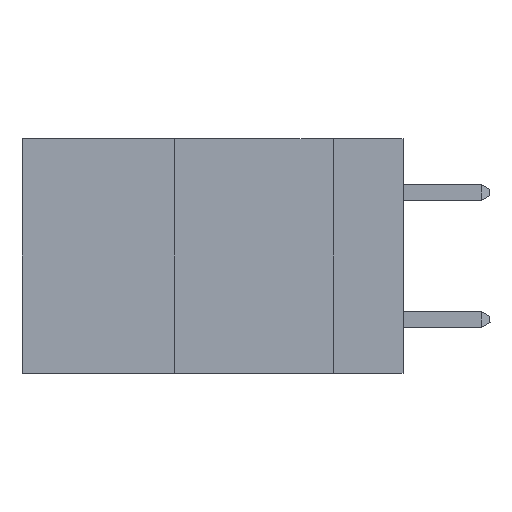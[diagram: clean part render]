
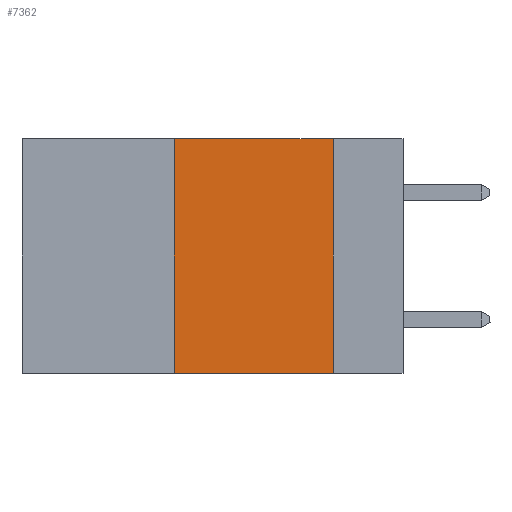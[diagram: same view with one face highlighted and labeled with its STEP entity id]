
A CAD part, left-side view. The second image highlights one B-rep face of the part: STEP entity #7362.
In plain terms, the highlighted planar face has unit normal (-1, 0, 0).
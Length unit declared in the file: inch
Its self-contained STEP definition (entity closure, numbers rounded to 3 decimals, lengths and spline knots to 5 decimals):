
#222 = VERTEX_POINT ( 'NONE', #383 ) ;
#383 = CARTESIAN_POINT ( 'NONE',  ( 0., 0.36, -0.37 ) ) ;
#716 = DIRECTION ( 'NONE',  ( 0., 0., -1. ) ) ;
#1097 = DIRECTION ( 'NONE',  ( 0., 0., 1. ) ) ;
#1168 = VECTOR ( 'NONE', #9938, 39.37008 ) ;
#2051 = CARTESIAN_POINT ( 'NONE',  ( 0., 0.36, 0. ) ) ;
#2286 = CARTESIAN_POINT ( 'NONE',  ( 0., 0.36, 0. ) ) ;
#2443 = EDGE_CURVE ( 'NONE', #222, #6811, #13166, .T. ) ;
#3015 = EDGE_LOOP ( 'NONE', ( #5993, #12001, #3783, #4115 ) ) ;
#3783 = ORIENTED_EDGE ( 'NONE', *, *, #2443, .F. ) ;
#4115 = ORIENTED_EDGE ( 'NONE', *, *, #9766, .T. ) ;
#4386 = LINE ( 'NONE', #5401, #6922 ) ;
#4766 = FACE_OUTER_BOUND ( 'NONE', #3015, .T. ) ;
#5401 = CARTESIAN_POINT ( 'NONE',  ( 0., 0.6, -0.37 ) ) ;
#5694 = CARTESIAN_POINT ( 'NONE',  ( 0., 0.6, 0. ) ) ;
#5993 = ORIENTED_EDGE ( 'NONE', *, *, #7477, .F. ) ;
#6811 = VERTEX_POINT ( 'NONE', #2051 ) ;
#6922 = VECTOR ( 'NONE', #13944, 39.37008 ) ;
#7355 = DIRECTION ( 'NONE',  ( 1., 0., 0. ) ) ;
#7362 = ADVANCED_FACE ( 'NONE', ( #4766 ), #12680, .F. ) ;
#7378 = CARTESIAN_POINT ( 'NONE',  ( 0., 0.11, -0.37 ) ) ;
#7424 = AXIS2_PLACEMENT_3D ( 'NONE', #10515, #7355, #716 ) ;
#7477 = EDGE_CURVE ( 'NONE', #9515, #9173, #8145, .T. ) ;
#7550 = CARTESIAN_POINT ( 'NONE',  ( 0., 0.11, 0. ) ) ;
#8145 = LINE ( 'NONE', #7550, #13494 ) ;
#8612 = DIRECTION ( 'NONE',  ( 0., 0., -1. ) ) ;
#9173 = VERTEX_POINT ( 'NONE', #7378 ) ;
#9515 = VERTEX_POINT ( 'NONE', #10343 ) ;
#9766 = EDGE_CURVE ( 'NONE', #222, #9173, #4386, .T. ) ;
#9881 = LINE ( 'NONE', #5694, #1168 ) ;
#9938 = DIRECTION ( 'NONE',  ( 0., -1., 0. ) ) ;
#10295 = VECTOR ( 'NONE', #1097, 39.37008 ) ;
#10343 = CARTESIAN_POINT ( 'NONE',  ( 0., 0.11, 0. ) ) ;
#10515 = CARTESIAN_POINT ( 'NONE',  ( 0., 0.6, 0. ) ) ;
#11256 = EDGE_CURVE ( 'NONE', #6811, #9515, #9881, .T. ) ;
#12001 = ORIENTED_EDGE ( 'NONE', *, *, #11256, .F. ) ;
#12680 = PLANE ( 'NONE',  #7424 ) ;
#13166 = LINE ( 'NONE', #2286, #10295 ) ;
#13494 = VECTOR ( 'NONE', #8612, 39.37008 ) ;
#13944 = DIRECTION ( 'NONE',  ( 0., -1., 0. ) ) ;
